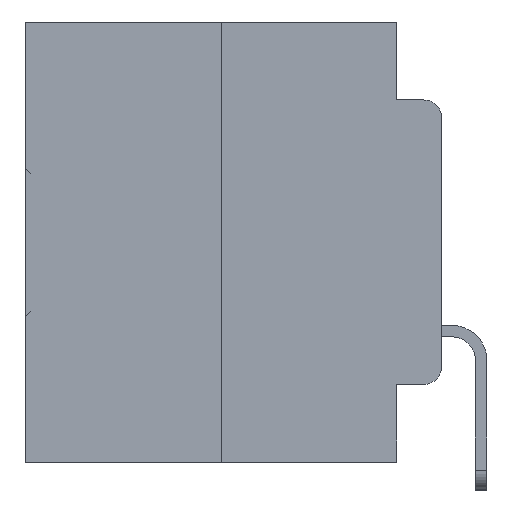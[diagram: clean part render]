
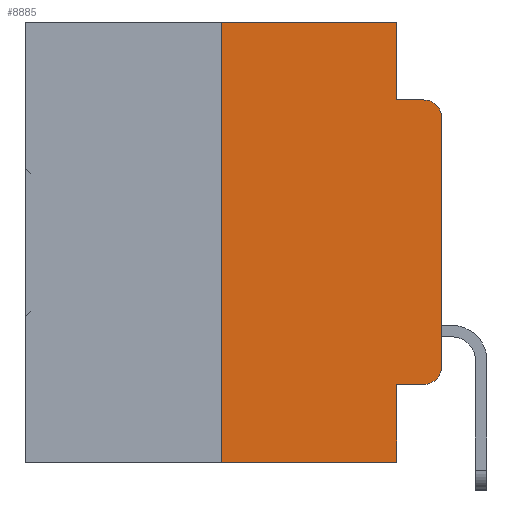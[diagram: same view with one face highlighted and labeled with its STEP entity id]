
A CAD part, left-side view. The second image highlights one B-rep face of the part: STEP entity #8885.
In plain terms, the highlighted planar face has unit normal (-1, 0, 0).
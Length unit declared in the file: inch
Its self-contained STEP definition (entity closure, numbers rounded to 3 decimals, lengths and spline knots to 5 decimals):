
#50 = DIRECTION ( 'NONE',  ( 0., 0., -1. ) ) ;
#1684 = VECTOR ( 'NONE', #21416, 39.37008 ) ;
#2158 = VERTEX_POINT ( 'NONE', #12496 ) ;
#2219 = CARTESIAN_POINT ( 'NONE',  ( 0., 0.051, -0.4115 ) ) ;
#2428 = DIRECTION ( 'NONE',  ( 0., 0., 1. ) ) ;
#2556 = LINE ( 'NONE', #8270, #1684 ) ;
#3357 = FACE_OUTER_BOUND ( 'NONE', #8065, .T. ) ;
#3431 = CARTESIAN_POINT ( 'NONE',  ( 0., 0.02, -0.4115 ) ) ;
#3773 = AXIS2_PLACEMENT_3D ( 'NONE', #14874, #31848, #17522 ) ;
#4120 = DIRECTION ( 'NONE',  ( -1., 0., 0. ) ) ;
#4193 = EDGE_CURVE ( 'NONE', #16475, #12440, #26182, .T. ) ;
#4465 = CARTESIAN_POINT ( 'NONE',  ( 0., 0.051, 0. ) ) ;
#5539 = VECTOR ( 'NONE', #25847, 39.37008 ) ;
#6056 = CARTESIAN_POINT ( 'NONE',  ( 0., 0.051, -0.0885 ) ) ;
#6305 = EDGE_CURVE ( 'NONE', #21025, #2158, #2556, .T. ) ;
#6992 = VECTOR ( 'NONE', #18688, 39.37008 ) ;
#7254 = VERTEX_POINT ( 'NONE', #3431 ) ;
#7834 = CARTESIAN_POINT ( 'NONE',  ( 0., 0.473, 0. ) ) ;
#8065 = EDGE_LOOP ( 'NONE', ( #14297, #15972, #16796, #12234, #25694, #20036, #32541, #13911, #21558, #8363 ) ) ;
#8270 = CARTESIAN_POINT ( 'NONE',  ( 0., 0.473, -0.5 ) ) ;
#8363 = ORIENTED_EDGE ( 'NONE', *, *, #17336, .T. ) ;
#8560 = LINE ( 'NONE', #2219, #14941 ) ;
#8885 = ADVANCED_FACE ( 'NONE', ( #3357 ), #12169, .F. ) ;
#9471 = VECTOR ( 'NONE', #20564, 39.37008 ) ;
#10824 = CIRCLE ( 'NONE', #30608, 0.02 ) ;
#11444 = CARTESIAN_POINT ( 'NONE',  ( 0., 0.051, 0. ) ) ;
#12169 = PLANE ( 'NONE',  #3773 ) ;
#12234 = ORIENTED_EDGE ( 'NONE', *, *, #16702, .F. ) ;
#12239 = CARTESIAN_POINT ( 'NONE',  ( 0., 0.051, -0.0885 ) ) ;
#12440 = VERTEX_POINT ( 'NONE', #11444 ) ;
#12451 = LINE ( 'NONE', #21078, #18664 ) ;
#12496 = CARTESIAN_POINT ( 'NONE',  ( 0., 0.051, -0.5 ) ) ;
#13190 = DIRECTION ( 'NONE',  ( 0., -1., 0. ) ) ;
#13395 = DIRECTION ( 'NONE',  ( 0., 0., -1. ) ) ;
#13495 = VERTEX_POINT ( 'NONE', #6056 ) ;
#13911 = ORIENTED_EDGE ( 'NONE', *, *, #16815, .F. ) ;
#14297 = ORIENTED_EDGE ( 'NONE', *, *, #14373, .T. ) ;
#14373 = EDGE_CURVE ( 'NONE', #18229, #18855, #32778, .T. ) ;
#14429 = EDGE_CURVE ( 'NONE', #18855, #27199, #10824, .T. ) ;
#14874 = CARTESIAN_POINT ( 'NONE',  ( 0., 0.473, 0. ) ) ;
#14941 = VECTOR ( 'NONE', #13190, 39.37008 ) ;
#15116 = CIRCLE ( 'NONE', #18690, 0.02 ) ;
#15903 = CARTESIAN_POINT ( 'NONE',  ( 0., 0., -0.1085 ) ) ;
#15972 = ORIENTED_EDGE ( 'NONE', *, *, #14429, .T. ) ;
#16379 = DIRECTION ( 'NONE',  ( -1., 0., 0. ) ) ;
#16475 = VERTEX_POINT ( 'NONE', #19374 ) ;
#16603 = EDGE_CURVE ( 'NONE', #13495, #27199, #27765, .T. ) ;
#16614 = LINE ( 'NONE', #4465, #9471 ) ;
#16702 = EDGE_CURVE ( 'NONE', #12440, #13495, #16614, .T. ) ;
#16755 = CARTESIAN_POINT ( 'NONE',  ( 0., 0.25, -0.5 ) ) ;
#16796 = ORIENTED_EDGE ( 'NONE', *, *, #16603, .F. ) ;
#16806 = EDGE_CURVE ( 'NONE', #21025, #16475, #19443, .T. ) ;
#16815 = EDGE_CURVE ( 'NONE', #19190, #2158, #12451, .T. ) ;
#17065 = EDGE_CURVE ( 'NONE', #19190, #7254, #8560, .T. ) ;
#17336 = EDGE_CURVE ( 'NONE', #7254, #18229, #15116, .T. ) ;
#17522 = DIRECTION ( 'NONE',  ( 0., 0., -1. ) ) ;
#17595 = DIRECTION ( 'NONE',  ( 0., -1., 0. ) ) ;
#18229 = VERTEX_POINT ( 'NONE', #19306 ) ;
#18590 = CARTESIAN_POINT ( 'NONE',  ( 0., 0.25, 0. ) ) ;
#18664 = VECTOR ( 'NONE', #13395, 39.37008 ) ;
#18688 = DIRECTION ( 'NONE',  ( 0., 0., 1. ) ) ;
#18690 = AXIS2_PLACEMENT_3D ( 'NONE', #20145, #4120, #22593 ) ;
#18855 = VERTEX_POINT ( 'NONE', #15903 ) ;
#19190 = VERTEX_POINT ( 'NONE', #31839 ) ;
#19306 = CARTESIAN_POINT ( 'NONE',  ( 0., 0., -0.3915 ) ) ;
#19374 = CARTESIAN_POINT ( 'NONE',  ( 0., 0.25, 0. ) ) ;
#19443 = LINE ( 'NONE', #18590, #32035 ) ;
#20036 = ORIENTED_EDGE ( 'NONE', *, *, #16806, .F. ) ;
#20145 = CARTESIAN_POINT ( 'NONE',  ( 0., 0.02, -0.3915 ) ) ;
#20564 = DIRECTION ( 'NONE',  ( 0., 0., -1. ) ) ;
#20627 = VECTOR ( 'NONE', #17595, 39.37008 ) ;
#21025 = VERTEX_POINT ( 'NONE', #16755 ) ;
#21078 = CARTESIAN_POINT ( 'NONE',  ( 0., 0.051, 0. ) ) ;
#21416 = DIRECTION ( 'NONE',  ( 0., -1., 0. ) ) ;
#21558 = ORIENTED_EDGE ( 'NONE', *, *, #17065, .T. ) ;
#22593 = DIRECTION ( 'NONE',  ( 0., 0., -1. ) ) ;
#25694 = ORIENTED_EDGE ( 'NONE', *, *, #4193, .F. ) ;
#25847 = DIRECTION ( 'NONE',  ( 0., -1., 0. ) ) ;
#26182 = LINE ( 'NONE', #7834, #5539 ) ;
#27199 = VERTEX_POINT ( 'NONE', #28466 ) ;
#27765 = LINE ( 'NONE', #12239, #20627 ) ;
#28466 = CARTESIAN_POINT ( 'NONE',  ( 0., 0.02, -0.0885 ) ) ;
#30608 = AXIS2_PLACEMENT_3D ( 'NONE', #30859, #16379, #50 ) ;
#30859 = CARTESIAN_POINT ( 'NONE',  ( 0., 0.02, -0.1085 ) ) ;
#31839 = CARTESIAN_POINT ( 'NONE',  ( 0., 0.051, -0.4115 ) ) ;
#31848 = DIRECTION ( 'NONE',  ( 1., 0., 0. ) ) ;
#32035 = VECTOR ( 'NONE', #2428, 39.37008 ) ;
#32541 = ORIENTED_EDGE ( 'NONE', *, *, #6305, .T. ) ;
#32778 = LINE ( 'NONE', #32826, #6992 ) ;
#32826 = CARTESIAN_POINT ( 'NONE',  ( 0., 0., 0. ) ) ;
